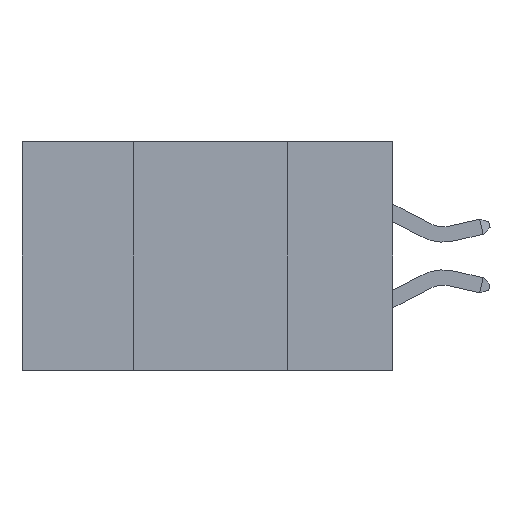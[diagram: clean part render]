
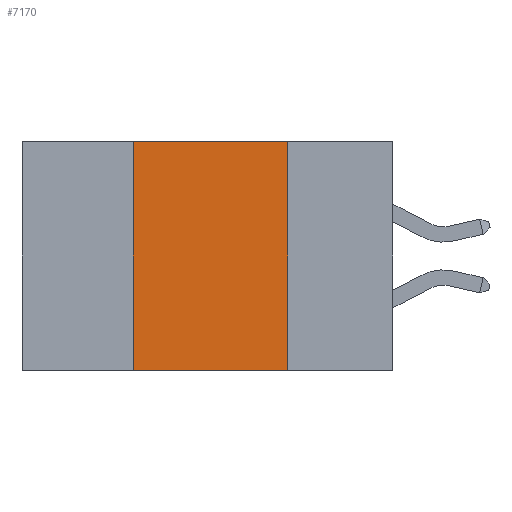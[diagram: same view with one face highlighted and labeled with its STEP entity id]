
A CAD part, left-side view. The second image highlights one B-rep face of the part: STEP entity #7170.
In plain terms, the highlighted planar face has unit normal (-1, 0, 0).
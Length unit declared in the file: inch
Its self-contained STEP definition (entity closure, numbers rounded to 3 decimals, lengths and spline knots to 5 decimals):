
#624 = EDGE_CURVE ( 'NONE', #4464, #5403, #9854, .T. ) ;
#781 = CARTESIAN_POINT ( 'NONE',  ( 0., 0.17, 0. ) ) ;
#885 = CARTESIAN_POINT ( 'NONE',  ( 0., 0.6, 0. ) ) ;
#1613 = ORIENTED_EDGE ( 'NONE', *, *, #624, .F. ) ;
#1768 = CARTESIAN_POINT ( 'NONE',  ( 0., 0.42, -0.37 ) ) ;
#2013 = EDGE_CURVE ( 'NONE', #5400, #10057, #8218, .T. ) ;
#2423 = ORIENTED_EDGE ( 'NONE', *, *, #10994, .F. ) ;
#2453 = CARTESIAN_POINT ( 'NONE',  ( 0., 0.17, -0.37 ) ) ;
#2666 = LINE ( 'NONE', #11442, #12570 ) ;
#3129 = CARTESIAN_POINT ( 'NONE',  ( 0., 0.42, 0. ) ) ;
#3916 = DIRECTION ( 'NONE',  ( 0., 0., -1. ) ) ;
#4464 = VERTEX_POINT ( 'NONE', #8673 ) ;
#4771 = CARTESIAN_POINT ( 'NONE',  ( 0., 0.6, 0. ) ) ;
#4884 = DIRECTION ( 'NONE',  ( 0., -1., 0. ) ) ;
#4957 = PLANE ( 'NONE',  #10271 ) ;
#5367 = ORIENTED_EDGE ( 'NONE', *, *, #10877, .F. ) ;
#5400 = VERTEX_POINT ( 'NONE', #1768 ) ;
#5403 = VERTEX_POINT ( 'NONE', #781 ) ;
#6147 = DIRECTION ( 'NONE',  ( 0., 0., 1. ) ) ;
#7170 = ADVANCED_FACE ( 'NONE', ( #8948 ), #4957, .F. ) ;
#7241 = DIRECTION ( 'NONE',  ( 0., -1., 0. ) ) ;
#7432 = VECTOR ( 'NONE', #6147, 39.37008 ) ;
#8218 = LINE ( 'NONE', #9258, #10727 ) ;
#8540 = ORIENTED_EDGE ( 'NONE', *, *, #2013, .T. ) ;
#8673 = CARTESIAN_POINT ( 'NONE',  ( 0., 0.42, 0. ) ) ;
#8948 = FACE_OUTER_BOUND ( 'NONE', #10778, .T. ) ;
#9258 = CARTESIAN_POINT ( 'NONE',  ( 0., 0.6, -0.37 ) ) ;
#9508 = VECTOR ( 'NONE', #4884, 39.37008 ) ;
#9532 = DIRECTION ( 'NONE',  ( 0., 0., -1. ) ) ;
#9854 = LINE ( 'NONE', #885, #9508 ) ;
#10057 = VERTEX_POINT ( 'NONE', #2453 ) ;
#10271 = AXIS2_PLACEMENT_3D ( 'NONE', #4771, #10786, #3916 ) ;
#10727 = VECTOR ( 'NONE', #7241, 39.37008 ) ;
#10778 = EDGE_LOOP ( 'NONE', ( #2423, #1613, #5367, #8540 ) ) ;
#10786 = DIRECTION ( 'NONE',  ( 1., 0., 0. ) ) ;
#10877 = EDGE_CURVE ( 'NONE', #5400, #4464, #11117, .T. ) ;
#10994 = EDGE_CURVE ( 'NONE', #5403, #10057, #2666, .T. ) ;
#11117 = LINE ( 'NONE', #3129, #7432 ) ;
#11442 = CARTESIAN_POINT ( 'NONE',  ( 0., 0.17, 0. ) ) ;
#12570 = VECTOR ( 'NONE', #9532, 39.37008 ) ;
